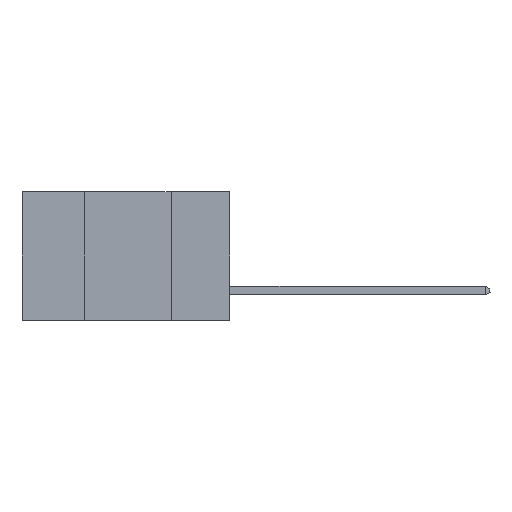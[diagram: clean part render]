
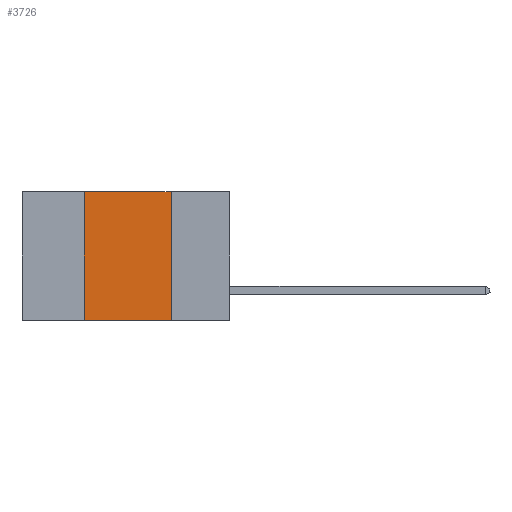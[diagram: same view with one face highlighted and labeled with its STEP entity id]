
A CAD part, left-side view. The second image highlights one B-rep face of the part: STEP entity #3726.
In plain terms, the highlighted planar face has unit normal (-1, 0, 0).
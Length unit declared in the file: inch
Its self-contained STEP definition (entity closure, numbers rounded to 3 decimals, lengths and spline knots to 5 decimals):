
#252 = CARTESIAN_POINT ( 'NONE',  ( 0., 0.42, 0. ) ) ;
#604 = VERTEX_POINT ( 'NONE', #252 ) ;
#922 = LINE ( 'NONE', #1811, #11993 ) ;
#1369 = DIRECTION ( 'NONE',  ( 0., 0., -1. ) ) ;
#1811 = CARTESIAN_POINT ( 'NONE',  ( 0., 0.42, 0. ) ) ;
#2224 = CARTESIAN_POINT ( 'NONE',  ( 0., 0.6, 0. ) ) ;
#2568 = LINE ( 'NONE', #9921, #5469 ) ;
#2687 = CARTESIAN_POINT ( 'NONE',  ( 0., 0.17, -0.37 ) ) ;
#2805 = VECTOR ( 'NONE', #4994, 39.37008 ) ;
#2830 = EDGE_CURVE ( 'NONE', #604, #6184, #7382, .T. ) ;
#3118 = CARTESIAN_POINT ( 'NONE',  ( 0., 0.42, -0.37 ) ) ;
#3726 = ADVANCED_FACE ( 'NONE', ( #8276 ), #12139, .F. ) ;
#3973 = EDGE_LOOP ( 'NONE', ( #11609, #10710, #7386, #7619 ) ) ;
#4994 = DIRECTION ( 'NONE',  ( 0., -1., 0. ) ) ;
#5469 = VECTOR ( 'NONE', #6019, 39.37008 ) ;
#6019 = DIRECTION ( 'NONE',  ( 0., -1., 0. ) ) ;
#6150 = LINE ( 'NONE', #7742, #9229 ) ;
#6184 = VERTEX_POINT ( 'NONE', #8921 ) ;
#6245 = DIRECTION ( 'NONE',  ( 1., 0., 0. ) ) ;
#6363 = EDGE_CURVE ( 'NONE', #8453, #8691, #2568, .T. ) ;
#7382 = LINE ( 'NONE', #8501, #2805 ) ;
#7386 = ORIENTED_EDGE ( 'NONE', *, *, #9156, .F. ) ;
#7619 = ORIENTED_EDGE ( 'NONE', *, *, #6363, .T. ) ;
#7742 = CARTESIAN_POINT ( 'NONE',  ( 0., 0.17, 0. ) ) ;
#8276 = FACE_OUTER_BOUND ( 'NONE', #3973, .T. ) ;
#8453 = VERTEX_POINT ( 'NONE', #3118 ) ;
#8501 = CARTESIAN_POINT ( 'NONE',  ( 0., 0.6, 0. ) ) ;
#8691 = VERTEX_POINT ( 'NONE', #2687 ) ;
#8845 = AXIS2_PLACEMENT_3D ( 'NONE', #2224, #6245, #1369 ) ;
#8921 = CARTESIAN_POINT ( 'NONE',  ( 0., 0.17, 0. ) ) ;
#9142 = EDGE_CURVE ( 'NONE', #6184, #8691, #6150, .T. ) ;
#9156 = EDGE_CURVE ( 'NONE', #8453, #604, #922, .T. ) ;
#9229 = VECTOR ( 'NONE', #10719, 39.37008 ) ;
#9724 = DIRECTION ( 'NONE',  ( 0., 0., 1. ) ) ;
#9921 = CARTESIAN_POINT ( 'NONE',  ( 0., 0.6, -0.37 ) ) ;
#10710 = ORIENTED_EDGE ( 'NONE', *, *, #2830, .F. ) ;
#10719 = DIRECTION ( 'NONE',  ( 0., 0., -1. ) ) ;
#11609 = ORIENTED_EDGE ( 'NONE', *, *, #9142, .F. ) ;
#11993 = VECTOR ( 'NONE', #9724, 39.37008 ) ;
#12139 = PLANE ( 'NONE',  #8845 ) ;
